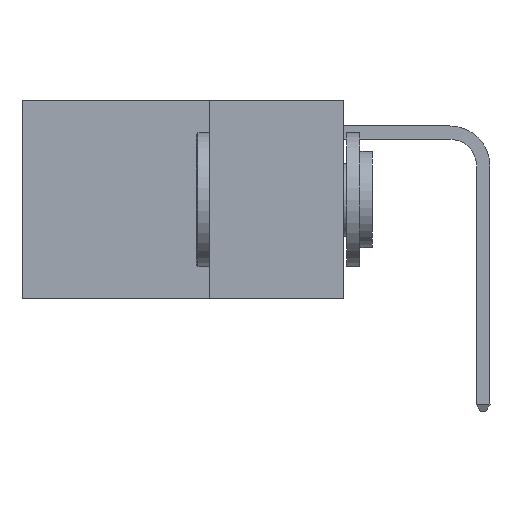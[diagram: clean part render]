
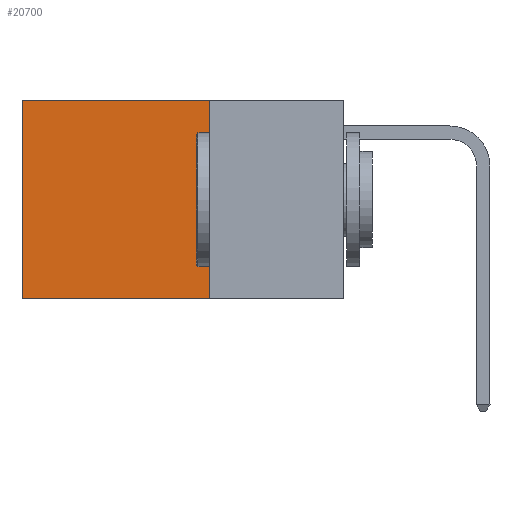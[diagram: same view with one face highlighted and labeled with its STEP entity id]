
A CAD part, left-side view. The second image highlights one B-rep face of the part: STEP entity #20700.
In plain terms, the highlighted planar face has unit normal (-1, 0, 0).
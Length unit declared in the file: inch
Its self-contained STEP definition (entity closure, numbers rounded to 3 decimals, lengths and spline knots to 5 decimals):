
#406 = DIRECTION ( 'NONE',  ( 0., 1., 0. ) ) ;
#820 = LINE ( 'NONE', #6560, #23118 ) ;
#1027 = CARTESIAN_POINT ( 'NONE',  ( 0.2625, 0.25, 0. ) ) ;
#1474 = EDGE_LOOP ( 'NONE', ( #9499, #11840, #17404, #4358 ) ) ;
#4358 = ORIENTED_EDGE ( 'NONE', *, *, #8530, .T. ) ;
#5528 = VECTOR ( 'NONE', #9329, 39.37008 ) ;
#5766 = CARTESIAN_POINT ( 'NONE',  ( 0.2625, 0.25, -0.37 ) ) ;
#5843 = PLANE ( 'NONE',  #20490 ) ;
#6560 = CARTESIAN_POINT ( 'NONE',  ( 0.2625, 0.25, 0. ) ) ;
#6943 = DIRECTION ( 'NONE',  ( 0., 0., -1. ) ) ;
#7529 = CARTESIAN_POINT ( 'NONE',  ( 0.2625, 0.6, 0. ) ) ;
#7684 = CARTESIAN_POINT ( 'NONE',  ( 0.2625, 0.25, 0. ) ) ;
#8530 = EDGE_CURVE ( 'NONE', #11653, #18499, #14067, .T. ) ;
#9204 = VECTOR ( 'NONE', #406, 39.37008 ) ;
#9329 = DIRECTION ( 'NONE',  ( 0., 0., -1. ) ) ;
#9499 = ORIENTED_EDGE ( 'NONE', *, *, #23372, .T. ) ;
#10364 = LINE ( 'NONE', #7529, #5528 ) ;
#10487 = LINE ( 'NONE', #23192, #20000 ) ;
#11336 = DIRECTION ( 'NONE',  ( 0., 0., -1. ) ) ;
#11653 = VERTEX_POINT ( 'NONE', #15310 ) ;
#11840 = ORIENTED_EDGE ( 'NONE', *, *, #21166, .F. ) ;
#12824 = EDGE_CURVE ( 'NONE', #11653, #23409, #820, .T. ) ;
#13219 = CARTESIAN_POINT ( 'NONE',  ( 0.2625, 0.6, -0.37 ) ) ;
#13416 = CARTESIAN_POINT ( 'NONE',  ( 0.2625, 0.6, 0. ) ) ;
#14067 = LINE ( 'NONE', #1027, #9204 ) ;
#14318 = VERTEX_POINT ( 'NONE', #13219 ) ;
#15310 = CARTESIAN_POINT ( 'NONE',  ( 0.2625, 0.25, 0. ) ) ;
#16118 = DIRECTION ( 'NONE',  ( 0., 1., 0. ) ) ;
#17404 = ORIENTED_EDGE ( 'NONE', *, *, #12824, .F. ) ;
#18499 = VERTEX_POINT ( 'NONE', #13416 ) ;
#19474 = FACE_OUTER_BOUND ( 'NONE', #1474, .T. ) ;
#20000 = VECTOR ( 'NONE', #16118, 39.37008 ) ;
#20490 = AXIS2_PLACEMENT_3D ( 'NONE', #7684, #21965, #11336 ) ;
#20700 = ADVANCED_FACE ( 'NONE', ( #19474 ), #5843, .F. ) ;
#21166 = EDGE_CURVE ( 'NONE', #23409, #14318, #10487, .T. ) ;
#21965 = DIRECTION ( 'NONE',  ( 1., 0., 0. ) ) ;
#23118 = VECTOR ( 'NONE', #6943, 39.37008 ) ;
#23192 = CARTESIAN_POINT ( 'NONE',  ( 0.2625, 0.25, -0.37 ) ) ;
#23372 = EDGE_CURVE ( 'NONE', #18499, #14318, #10364, .T. ) ;
#23409 = VERTEX_POINT ( 'NONE', #5766 ) ;
